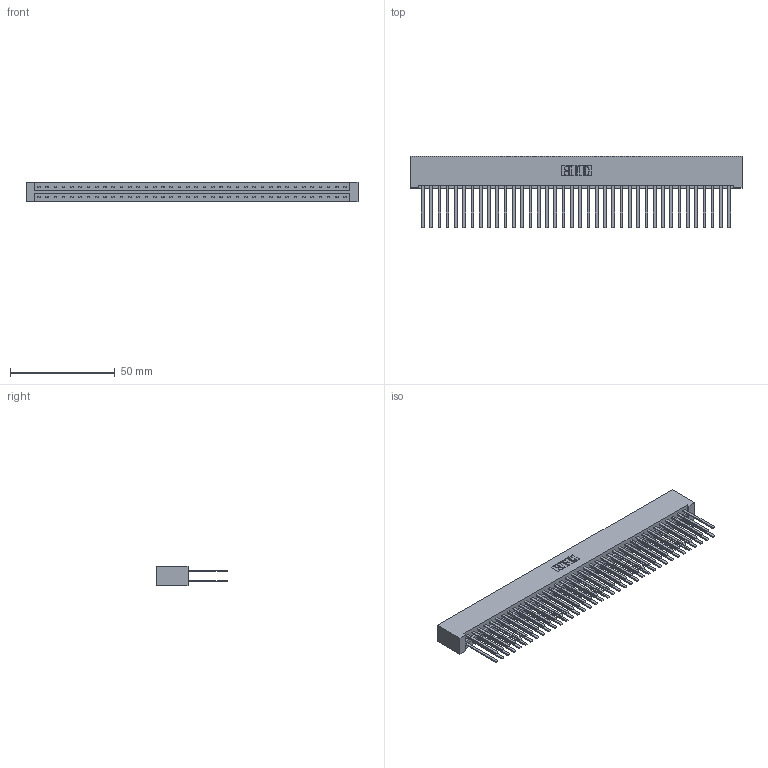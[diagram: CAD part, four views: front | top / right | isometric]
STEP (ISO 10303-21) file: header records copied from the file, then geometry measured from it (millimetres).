
FILE_DESCRIPTION (( 'STEP AP203' ), '1' );
FILE_NAME ('333-076-544-201.STEP', '2018-08-04T23:13:21', ( '' ), ( '' ), 'SwSTEP 2.0', 'SolidWorks 2016', '' );
FILE_SCHEMA (( 'CONFIG_CONTROL_DESIGN' ));
Length unit declared in the file: inch
Products named in the file (3): 333 Part_Lugless; 345-292-001_345-293-144; 333-076-544-201
Assembly tree (77 placements, depth 2):
  333-076-544-201
    333 Part_Lugless
    345-292-001_345-293-144  x76
Bounding box: 158.83 x 34.3 x 9.4 mm (x, y, z)
Volume: 17875.4 mm3; surface area: 24544.9 mm2
Topology: 77 solids, 77 shells, 3602 faces, 10699 edges, 7030 vertices
Faces by surface type: plane 2498, cylinder 1104
Entity records: 24503 total; most frequent: CARTESIAN_POINT 4062, ORIENTED_EDGE 3998, DIRECTION 3467, EDGE_CURVE 1999, VECTOR 1883, LINE 1883, VERTEX_POINT 1330, AXIS2_PLACEMENT_3D 792
